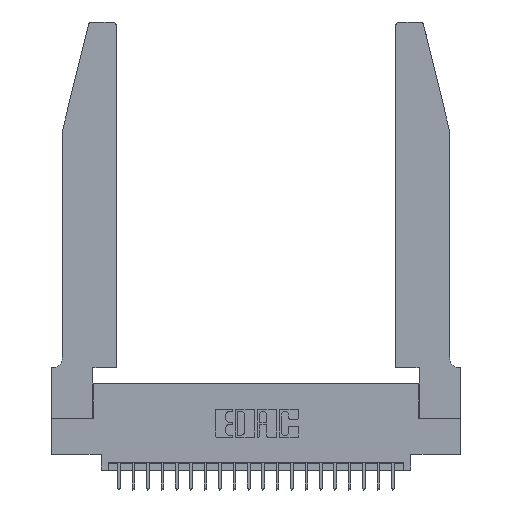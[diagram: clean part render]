
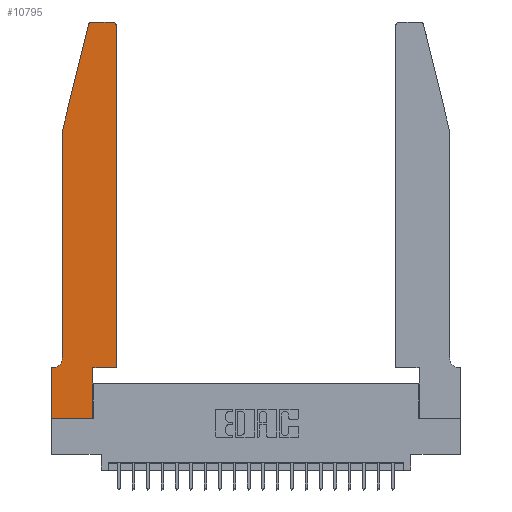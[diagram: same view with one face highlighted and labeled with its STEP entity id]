
A CAD part, top view. The second image highlights one B-rep face of the part: STEP entity #10795.
In plain terms, the highlighted planar face has unit normal (0, 0, 1).
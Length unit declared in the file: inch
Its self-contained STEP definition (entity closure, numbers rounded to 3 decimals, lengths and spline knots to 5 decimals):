
#6 = VECTOR ( 'NONE', #7278, 39.37008 ) ;
#104 = CIRCLE ( 'NONE', #21917, 0.03 ) ;
#579 = ORIENTED_EDGE ( 'NONE', *, *, #20629, .T. ) ;
#601 = VERTEX_POINT ( 'NONE', #9388 ) ;
#1148 = CARTESIAN_POINT ( 'NONE',  ( 0.25487, 2.72718, 0.37 ) ) ;
#1577 = CARTESIAN_POINT ( 'NONE',  ( 0.4505, 0.35, 0.37 ) ) ;
#1865 = LINE ( 'NONE', #23406, #4575 ) ;
#1918 = AXIS2_PLACEMENT_3D ( 'NONE', #17361, #17248, #23099 ) ;
#2226 = DIRECTION ( 'NONE',  ( 0., 1., 0. ) ) ;
#2278 = CARTESIAN_POINT ( 'NONE',  ( 0., 0., 0.37 ) ) ;
#2326 = LINE ( 'NONE', #13782, #20793 ) ;
#2486 = VERTEX_POINT ( 'NONE', #1577 ) ;
#2646 = VECTOR ( 'NONE', #7802, 39.37008 ) ;
#2823 = ORIENTED_EDGE ( 'NONE', *, *, #10118, .T. ) ;
#3854 = CARTESIAN_POINT ( 'NONE',  ( 0.0755, 2., 0.37 ) ) ;
#4038 = CARTESIAN_POINT ( 'NONE',  ( 0.4505, 0.35, 0.37 ) ) ;
#4482 = LINE ( 'NONE', #8219, #17360 ) ;
#4575 = VECTOR ( 'NONE', #9236, 39.37008 ) ;
#5347 = CIRCLE ( 'NONE', #7670, 0.03 ) ;
#5395 = VERTEX_POINT ( 'NONE', #11244 ) ;
#5585 = CARTESIAN_POINT ( 'NONE',  ( 0.2605, 2.75, 0.37 ) ) ;
#5657 = LINE ( 'NONE', #3854, #6238 ) ;
#5863 = ORIENTED_EDGE ( 'NONE', *, *, #13839, .T. ) ;
#5946 = ORIENTED_EDGE ( 'NONE', *, *, #9466, .T. ) ;
#6083 = CARTESIAN_POINT ( 'NONE',  ( 0.0755, 0.35, 0.37 ) ) ;
#6093 = CIRCLE ( 'NONE', #19455, 0.07 ) ;
#6238 = VECTOR ( 'NONE', #18424, 39.37008 ) ;
#6325 = VERTEX_POINT ( 'NONE', #13695 ) ;
#6680 = DIRECTION ( 'NONE',  ( -0.239, -0.971, 0. ) ) ;
#6880 = VERTEX_POINT ( 'NONE', #1148 ) ;
#6900 = DIRECTION ( 'NONE',  ( 1., 0., 0. ) ) ;
#6945 = EDGE_CURVE ( 'NONE', #10640, #8235, #6093, .T. ) ;
#7022 = EDGE_CURVE ( 'NONE', #13873, #5395, #1865, .T. ) ;
#7141 = EDGE_CURVE ( 'NONE', #8235, #601, #7547, .T. ) ;
#7278 = DIRECTION ( 'NONE',  ( -1., 0., 0. ) ) ;
#7547 = LINE ( 'NONE', #6083, #2646 ) ;
#7670 = AXIS2_PLACEMENT_3D ( 'NONE', #15958, #17990, #6900 ) ;
#7802 = DIRECTION ( 'NONE',  ( -1., 0., 0. ) ) ;
#7803 = DIRECTION ( 'NONE',  ( 0., 0., 1. ) ) ;
#8219 = CARTESIAN_POINT ( 'NONE',  ( 0.4505, 0.35, 0.37 ) ) ;
#8235 = VERTEX_POINT ( 'NONE', #20585 ) ;
#8933 = ORIENTED_EDGE ( 'NONE', *, *, #7022, .T. ) ;
#9138 = EDGE_CURVE ( 'NONE', #22802, #6880, #5347, .T. ) ;
#9236 = DIRECTION ( 'NONE',  ( 1., 0., 0. ) ) ;
#9388 = CARTESIAN_POINT ( 'NONE',  ( 0., 0.35, 0.37 ) ) ;
#9466 = EDGE_CURVE ( 'NONE', #601, #13873, #16975, .T. ) ;
#9545 = CARTESIAN_POINT ( 'NONE',  ( 0.0755, 2., 0.37 ) ) ;
#9831 = CARTESIAN_POINT ( 'NONE',  ( 0.4205, 2.75, 0.37 ) ) ;
#10024 = PLANE ( 'NONE',  #1918 ) ;
#10071 = ORIENTED_EDGE ( 'NONE', *, *, #15480, .T. ) ;
#10118 = EDGE_CURVE ( 'NONE', #2486, #19750, #22539, .T. ) ;
#10200 = ORIENTED_EDGE ( 'NONE', *, *, #7141, .T. ) ;
#10283 = CARTESIAN_POINT ( 'NONE',  ( 0.0755, 0.42, 0.37 ) ) ;
#10567 = EDGE_CURVE ( 'NONE', #14470, #22802, #16220, .T. ) ;
#10640 = VERTEX_POINT ( 'NONE', #10283 ) ;
#10795 = ADVANCED_FACE ( 'NONE', ( #19177 ), #10024, .T. ) ;
#11244 = CARTESIAN_POINT ( 'NONE',  ( 0.2865, 0., 0.37 ) ) ;
#11298 = ORIENTED_EDGE ( 'NONE', *, *, #14521, .T. ) ;
#12247 = CARTESIAN_POINT ( 'NONE',  ( 0.4505, 2.72, 0.37 ) ) ;
#12630 = VECTOR ( 'NONE', #22594, 39.37008 ) ;
#12907 = EDGE_LOOP ( 'NONE', ( #19548, #15493, #11298, #579, #15771, #10200, #5946, #8933, #15686, #10071, #2823, #5863 ) ) ;
#13695 = CARTESIAN_POINT ( 'NONE',  ( 0.2865, 0.35, 0.37 ) ) ;
#13782 = CARTESIAN_POINT ( 'NONE',  ( 0.2865, 0.35, 0.37 ) ) ;
#13839 = EDGE_CURVE ( 'NONE', #19750, #14470, #104, .T. ) ;
#13873 = VERTEX_POINT ( 'NONE', #15133 ) ;
#14229 = EDGE_CURVE ( 'NONE', #5395, #6325, #2326, .T. ) ;
#14470 = VERTEX_POINT ( 'NONE', #9831 ) ;
#14521 = EDGE_CURVE ( 'NONE', #6880, #16407, #20922, .T. ) ;
#14886 = DIRECTION ( 'NONE',  ( 0., 1., 0. ) ) ;
#15133 = CARTESIAN_POINT ( 'NONE',  ( 0., 0., 0.37 ) ) ;
#15445 = DIRECTION ( 'NONE',  ( 1., 0., 0. ) ) ;
#15480 = EDGE_CURVE ( 'NONE', #6325, #2486, #4482, .T. ) ;
#15493 = ORIENTED_EDGE ( 'NONE', *, *, #9138, .T. ) ;
#15686 = ORIENTED_EDGE ( 'NONE', *, *, #14229, .T. ) ;
#15771 = ORIENTED_EDGE ( 'NONE', *, *, #6945, .T. ) ;
#15958 = CARTESIAN_POINT ( 'NONE',  ( 0.284, 2.72, 0.37 ) ) ;
#16220 = LINE ( 'NONE', #5585, #6 ) ;
#16407 = VERTEX_POINT ( 'NONE', #9545 ) ;
#16722 = DIRECTION ( 'NONE',  ( 1., 0., 0. ) ) ;
#16975 = LINE ( 'NONE', #2278, #12630 ) ;
#17248 = DIRECTION ( 'NONE',  ( 0., 0., 1. ) ) ;
#17360 = VECTOR ( 'NONE', #15445, 39.37008 ) ;
#17361 = CARTESIAN_POINT ( 'NONE',  ( 0., 0.35, 0.37 ) ) ;
#17990 = DIRECTION ( 'NONE',  ( 0., 0., 1. ) ) ;
#18424 = DIRECTION ( 'NONE',  ( 0., -1., 0. ) ) ;
#18864 = CARTESIAN_POINT ( 'NONE',  ( 0.4205, 2.72, 0.37 ) ) ;
#19132 = DIRECTION ( 'NONE',  ( 0., 0., -1. ) ) ;
#19177 = FACE_OUTER_BOUND ( 'NONE', #12907, .T. ) ;
#19260 = VECTOR ( 'NONE', #6680, 39.37008 ) ;
#19455 = AXIS2_PLACEMENT_3D ( 'NONE', #21179, #19132, #20947 ) ;
#19548 = ORIENTED_EDGE ( 'NONE', *, *, #10567, .T. ) ;
#19750 = VERTEX_POINT ( 'NONE', #12247 ) ;
#20585 = CARTESIAN_POINT ( 'NONE',  ( 0.0055, 0.35, 0.37 ) ) ;
#20629 = EDGE_CURVE ( 'NONE', #16407, #10640, #5657, .T. ) ;
#20793 = VECTOR ( 'NONE', #14886, 39.37008 ) ;
#20922 = LINE ( 'NONE', #22333, #19260 ) ;
#20947 = DIRECTION ( 'NONE',  ( -1., 0., 0. ) ) ;
#21179 = CARTESIAN_POINT ( 'NONE',  ( 0.0055, 0.42, 0.37 ) ) ;
#21778 = VECTOR ( 'NONE', #2226, 39.37008 ) ;
#21917 = AXIS2_PLACEMENT_3D ( 'NONE', #18864, #7803, #16722 ) ;
#22333 = CARTESIAN_POINT ( 'NONE',  ( 0.0755, 2., 0.37 ) ) ;
#22539 = LINE ( 'NONE', #4038, #21778 ) ;
#22593 = CARTESIAN_POINT ( 'NONE',  ( 0.284, 2.75, 0.37 ) ) ;
#22594 = DIRECTION ( 'NONE',  ( 0., -1., 0. ) ) ;
#22802 = VERTEX_POINT ( 'NONE', #22593 ) ;
#23099 = DIRECTION ( 'NONE',  ( 1., 0., 0. ) ) ;
#23406 = CARTESIAN_POINT ( 'NONE',  ( 0., 0., 0.37 ) ) ;
